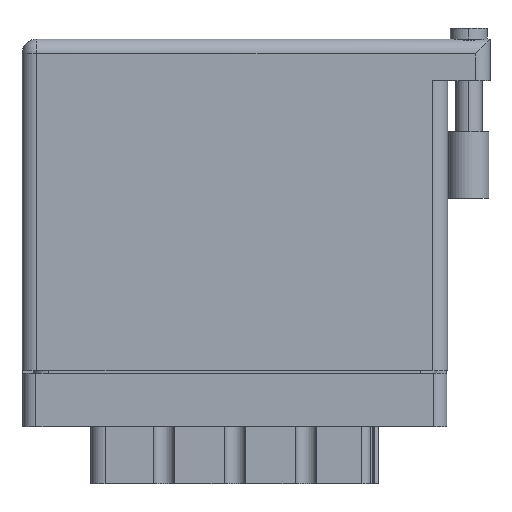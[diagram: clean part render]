
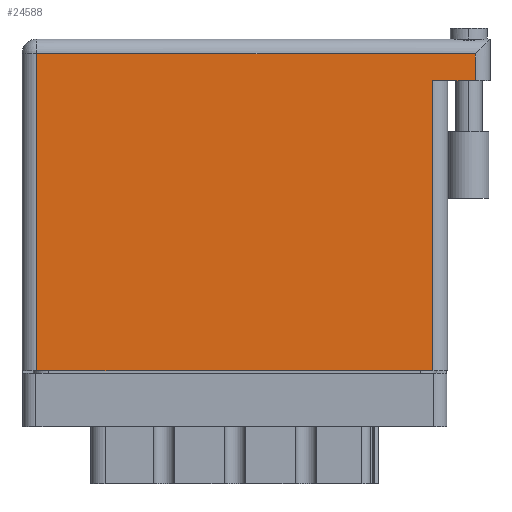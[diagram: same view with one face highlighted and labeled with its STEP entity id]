
A CAD part, front view. The second image highlights one B-rep face of the part: STEP entity #24588.
In plain terms, the highlighted face is planar.
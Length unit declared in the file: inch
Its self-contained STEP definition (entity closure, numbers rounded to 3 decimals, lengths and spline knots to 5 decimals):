
#1977 = VECTOR ( 'NONE', #13799, 39.37008 ) ;
#2293 = VERTEX_POINT ( 'NONE', #12139 ) ;
#3472 = CARTESIAN_POINT ( 'NONE',  ( 2.138, 1.496, 0. ) ) ;
#4393 = ORIENTED_EDGE ( 'NONE', *, *, #31324, .F. ) ;
#4707 = EDGE_CURVE ( 'NONE', #31602, #35605, #19294, .T. ) ;
#4953 = CARTESIAN_POINT ( 'NONE',  ( 1.938, 1.369, 0. ) ) ;
#5918 = FACE_OUTER_BOUND ( 'NONE', #30605, .T. ) ;
#6399 = CARTESIAN_POINT ( 'NONE',  ( 1.938, 1.369, 0. ) ) ;
#6717 = AXIS2_PLACEMENT_3D ( 'NONE', #28665, #25860, #15798 ) ;
#7917 = CARTESIAN_POINT ( 'NONE',  ( 2.138, 1.369, 0. ) ) ;
#8289 = DIRECTION ( 'NONE',  ( 0., 1., 0. ) ) ;
#9275 = CARTESIAN_POINT ( 'NONE',  ( 2.138, 1.566, 0. ) ) ;
#12139 = CARTESIAN_POINT ( 'NONE',  ( 0.07, 0., 0. ) ) ;
#13112 = EDGE_CURVE ( 'NONE', #26672, #15811, #22884, .T. ) ;
#13515 = LINE ( 'NONE', #33132, #24911 ) ;
#13660 = ORIENTED_EDGE ( 'NONE', *, *, #15707, .T. ) ;
#13776 = VECTOR ( 'NONE', #28296, 39.37008 ) ;
#13799 = DIRECTION ( 'NONE',  ( 0., -1., 0. ) ) ;
#15707 = EDGE_CURVE ( 'NONE', #30172, #26672, #32598, .T. ) ;
#15798 = DIRECTION ( 'NONE',  ( -1., 0., 0. ) ) ;
#15811 = VERTEX_POINT ( 'NONE', #18774 ) ;
#16174 = ORIENTED_EDGE ( 'NONE', *, *, #4707, .T. ) ;
#16189 = LINE ( 'NONE', #27568, #33869 ) ;
#17025 = CARTESIAN_POINT ( 'NONE',  ( 1.938, 0., 0. ) ) ;
#17281 = PLANE ( 'NONE',  #6717 ) ;
#18475 = EDGE_CURVE ( 'NONE', #2293, #31602, #16189, .T. ) ;
#18774 = CARTESIAN_POINT ( 'NONE',  ( 0.07, 1.496, 0. ) ) ;
#18956 = ORIENTED_EDGE ( 'NONE', *, *, #13112, .T. ) ;
#19108 = DIRECTION ( 'NONE',  ( -1., 0., 0. ) ) ;
#19171 = DIRECTION ( 'NONE',  ( 1., 0., 0. ) ) ;
#19294 = LINE ( 'NONE', #4953, #35298 ) ;
#21993 = LINE ( 'NONE', #25160, #1977 ) ;
#22884 = LINE ( 'NONE', #34286, #13776 ) ;
#24588 = ADVANCED_FACE ( 'NONE', ( #5918 ), #17281, .F. ) ;
#24911 = VECTOR ( 'NONE', #19108, 39.37008 ) ;
#25160 = CARTESIAN_POINT ( 'NONE',  ( 0.07, 0., 0. ) ) ;
#25860 = DIRECTION ( 'NONE',  ( 0., 0., -1. ) ) ;
#26021 = EDGE_CURVE ( 'NONE', #15811, #2293, #21993, .T. ) ;
#26330 = ORIENTED_EDGE ( 'NONE', *, *, #18475, .T. ) ;
#26672 = VERTEX_POINT ( 'NONE', #3472 ) ;
#27093 = ORIENTED_EDGE ( 'NONE', *, *, #26021, .T. ) ;
#27568 = CARTESIAN_POINT ( 'NONE',  ( 0., 0., 0. ) ) ;
#28296 = DIRECTION ( 'NONE',  ( -1., 0., 0. ) ) ;
#28319 = VECTOR ( 'NONE', #31854, 39.37008 ) ;
#28665 = CARTESIAN_POINT ( 'NONE',  ( 0., 1.566, 0. ) ) ;
#30172 = VERTEX_POINT ( 'NONE', #7917 ) ;
#30605 = EDGE_LOOP ( 'NONE', ( #26330, #16174, #4393, #13660, #18956, #27093 ) ) ;
#31324 = EDGE_CURVE ( 'NONE', #30172, #35605, #13515, .T. ) ;
#31602 = VERTEX_POINT ( 'NONE', #17025 ) ;
#31854 = DIRECTION ( 'NONE',  ( 0., 1., 0. ) ) ;
#32598 = LINE ( 'NONE', #9275, #28319 ) ;
#33132 = CARTESIAN_POINT ( 'NONE',  ( 2.208, 1.369, 0. ) ) ;
#33869 = VECTOR ( 'NONE', #19171, 39.37008 ) ;
#34286 = CARTESIAN_POINT ( 'NONE',  ( 0., 1.496, 0. ) ) ;
#35298 = VECTOR ( 'NONE', #8289, 39.37008 ) ;
#35605 = VERTEX_POINT ( 'NONE', #6399 ) ;
